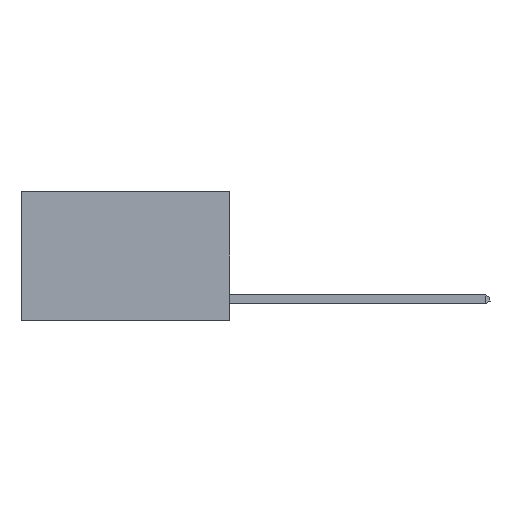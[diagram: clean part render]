
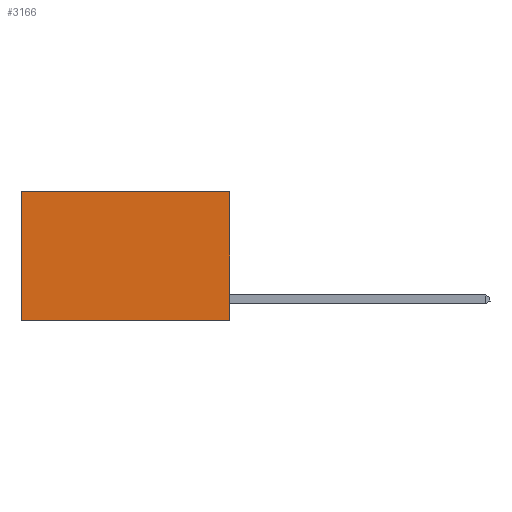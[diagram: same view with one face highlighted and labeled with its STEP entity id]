
A CAD part, left-side view. The second image highlights one B-rep face of the part: STEP entity #3166.
In plain terms, the highlighted planar face has unit normal (-1, 0, 0).
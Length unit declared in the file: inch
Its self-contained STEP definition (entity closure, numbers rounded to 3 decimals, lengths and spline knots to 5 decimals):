
#28 = VECTOR ( 'NONE', #18929, 39.37008 ) ;
#995 = ORIENTED_EDGE ( 'NONE', *, *, #17215, .F. ) ;
#1124 = DIRECTION ( 'NONE',  ( 0., 1., 0. ) ) ;
#2912 = VERTEX_POINT ( 'NONE', #3415 ) ;
#3166 = ADVANCED_FACE ( 'NONE', ( #14654 ), #6210, .F. ) ;
#3415 = CARTESIAN_POINT ( 'NONE',  ( 0.2625, 0., 0. ) ) ;
#3936 = ORIENTED_EDGE ( 'NONE', *, *, #15251, .T. ) ;
#4368 = CARTESIAN_POINT ( 'NONE',  ( 0.2625, 0., 0. ) ) ;
#4453 = CARTESIAN_POINT ( 'NONE',  ( 0.2625, 0., 0. ) ) ;
#5179 = LINE ( 'NONE', #20894, #14223 ) ;
#5507 = CARTESIAN_POINT ( 'NONE',  ( 0.2625, 0., 0. ) ) ;
#6210 = PLANE ( 'NONE',  #18690 ) ;
#6301 = VECTOR ( 'NONE', #7320, 39.37008 ) ;
#6693 = CARTESIAN_POINT ( 'NONE',  ( 0.2625, 0., -0.37 ) ) ;
#7320 = DIRECTION ( 'NONE',  ( 0., 0., -1. ) ) ;
#8022 = DIRECTION ( 'NONE',  ( 0., 0., -1. ) ) ;
#8578 = CARTESIAN_POINT ( 'NONE',  ( 0.2625, 0.6, 0. ) ) ;
#9223 = LINE ( 'NONE', #4453, #28 ) ;
#9340 = ORIENTED_EDGE ( 'NONE', *, *, #20284, .T. ) ;
#13489 = VERTEX_POINT ( 'NONE', #8578 ) ;
#14223 = VECTOR ( 'NONE', #22652, 39.37008 ) ;
#14654 = FACE_OUTER_BOUND ( 'NONE', #17900, .T. ) ;
#15251 = EDGE_CURVE ( 'NONE', #2912, #13489, #9223, .T. ) ;
#17215 = EDGE_CURVE ( 'NONE', #2912, #21004, #20654, .T. ) ;
#17701 = VERTEX_POINT ( 'NONE', #22887 ) ;
#17900 = EDGE_LOOP ( 'NONE', ( #9340, #19704, #995, #3936 ) ) ;
#18690 = AXIS2_PLACEMENT_3D ( 'NONE', #4368, #18849, #8022 ) ;
#18764 = LINE ( 'NONE', #6693, #22871 ) ;
#18849 = DIRECTION ( 'NONE',  ( 1., 0., 0. ) ) ;
#18929 = DIRECTION ( 'NONE',  ( 0., 1., 0. ) ) ;
#19196 = CARTESIAN_POINT ( 'NONE',  ( 0.2625, 0., -0.37 ) ) ;
#19704 = ORIENTED_EDGE ( 'NONE', *, *, #19719, .F. ) ;
#19719 = EDGE_CURVE ( 'NONE', #21004, #17701, #18764, .T. ) ;
#20284 = EDGE_CURVE ( 'NONE', #13489, #17701, #5179, .T. ) ;
#20654 = LINE ( 'NONE', #5507, #6301 ) ;
#20894 = CARTESIAN_POINT ( 'NONE',  ( 0.2625, 0.6, 0. ) ) ;
#21004 = VERTEX_POINT ( 'NONE', #19196 ) ;
#22652 = DIRECTION ( 'NONE',  ( 0., 0., -1. ) ) ;
#22871 = VECTOR ( 'NONE', #1124, 39.37008 ) ;
#22887 = CARTESIAN_POINT ( 'NONE',  ( 0.2625, 0.6, -0.37 ) ) ;
